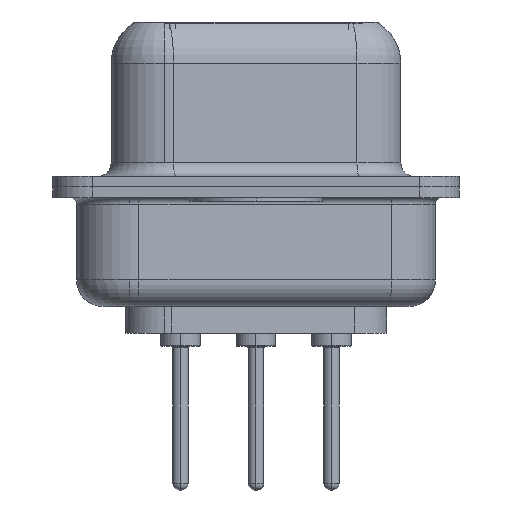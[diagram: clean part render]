
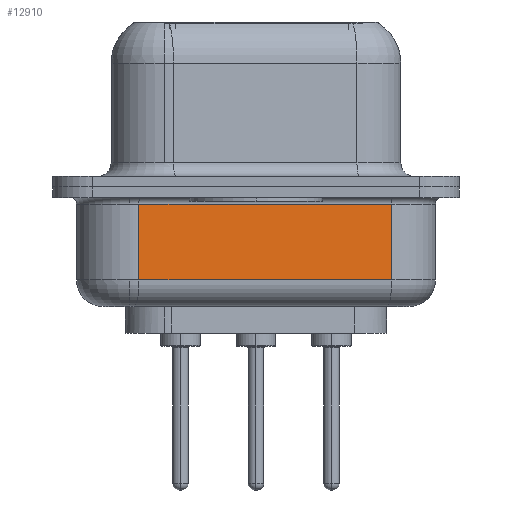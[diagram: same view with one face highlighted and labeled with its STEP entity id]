
A CAD part, left-side view. The second image highlights one B-rep face of the part: STEP entity #12910.
In plain terms, the highlighted planar face has unit normal (-0.985, -0.174, 0).
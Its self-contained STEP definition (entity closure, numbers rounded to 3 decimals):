
#1567 = DIRECTION ( 'NONE',  ( 0.985, 0.174, 0. ) ) ;
#2366 = ORIENTED_EDGE ( 'NONE', *, *, #5143, .F. ) ;
#2509 = LINE ( 'NONE', #17145, #2525 ) ;
#2525 = VECTOR ( 'NONE', #9747, 1000. ) ;
#2668 = VERTEX_POINT ( 'NONE', #16433 ) ;
#3980 = CARTESIAN_POINT ( 'NONE',  ( 2.93, 4.403, -0.65 ) ) ;
#4052 = EDGE_CURVE ( 'NONE', #2668, #25931, #26740, .T. ) ;
#5137 = CARTESIAN_POINT ( 'NONE',  ( 2.93, 4.403, -3.5 ) ) ;
#5141 = LINE ( 'NONE', #22312, #13329 ) ;
#5143 = EDGE_CURVE ( 'NONE', #2668, #11611, #5141, .T. ) ;
#5747 = LINE ( 'NONE', #22618, #8862 ) ;
#6451 = EDGE_CURVE ( 'NONE', #10999, #11611, #5747, .T. ) ;
#8862 = VECTOR ( 'NONE', #22133, 1000. ) ;
#8909 = ORIENTED_EDGE ( 'NONE', *, *, #4052, .T. ) ;
#9747 = DIRECTION ( 'NONE',  ( 0., 0., 1. ) ) ;
#10999 = VERTEX_POINT ( 'NONE', #17564 ) ;
#11451 = AXIS2_PLACEMENT_3D ( 'NONE', #28386, #1567, #30422 ) ;
#11611 = VERTEX_POINT ( 'NONE', #3980 ) ;
#12910 = ADVANCED_FACE ( 'NONE', ( #28070 ), #30748, .F. ) ;
#13329 = VECTOR ( 'NONE', #17256, 1000. ) ;
#14731 = DIRECTION ( 'NONE',  ( 0.174, -0.985, 0. ) ) ;
#16241 = ORIENTED_EDGE ( 'NONE', *, *, #6451, .T. ) ;
#16433 = CARTESIAN_POINT ( 'NONE',  ( 2.93, 4.403, -3.5 ) ) ;
#17145 = CARTESIAN_POINT ( 'NONE',  ( 4.605, -5.097, -4.5 ) ) ;
#17256 = DIRECTION ( 'NONE',  ( 0., 0., 1. ) ) ;
#17564 = CARTESIAN_POINT ( 'NONE',  ( 4.605, -5.097, -0.65 ) ) ;
#20710 = VECTOR ( 'NONE', #14731, 1000. ) ;
#22133 = DIRECTION ( 'NONE',  ( -0.174, 0.985, 0. ) ) ;
#22312 = CARTESIAN_POINT ( 'NONE',  ( 2.93, 4.403, -4.5 ) ) ;
#22618 = CARTESIAN_POINT ( 'NONE',  ( 2.93, 4.403, -0.65 ) ) ;
#25698 = EDGE_CURVE ( 'NONE', #25931, #10999, #2509, .T. ) ;
#25931 = VERTEX_POINT ( 'NONE', #26008 ) ;
#26008 = CARTESIAN_POINT ( 'NONE',  ( 4.605, -5.097, -3.5 ) ) ;
#26723 = EDGE_LOOP ( 'NONE', ( #2366, #8909, #29816, #16241 ) ) ;
#26740 = LINE ( 'NONE', #5137, #20710 ) ;
#28070 = FACE_OUTER_BOUND ( 'NONE', #26723, .T. ) ;
#28386 = CARTESIAN_POINT ( 'NONE',  ( 2.93, 4.403, -4.5 ) ) ;
#29816 = ORIENTED_EDGE ( 'NONE', *, *, #25698, .T. ) ;
#30422 = DIRECTION ( 'NONE',  ( -0.174, 0.985, 0. ) ) ;
#30748 = PLANE ( 'NONE',  #11451 ) ;
